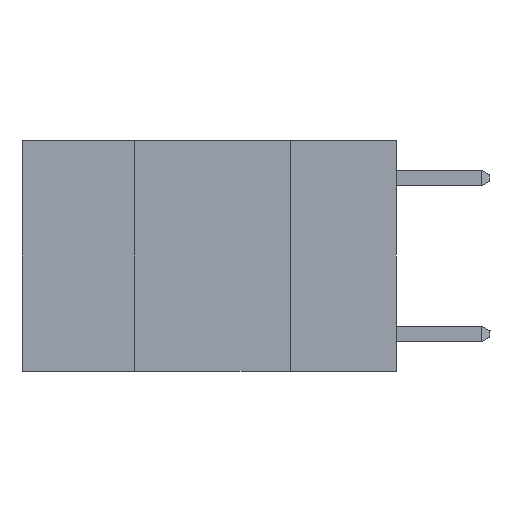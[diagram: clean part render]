
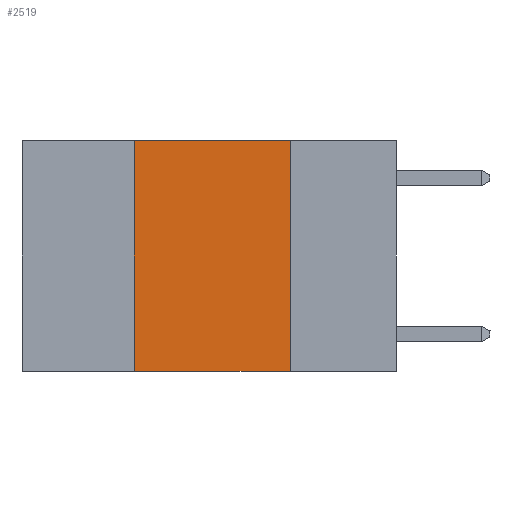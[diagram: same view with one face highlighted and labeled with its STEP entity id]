
A CAD part, left-side view. The second image highlights one B-rep face of the part: STEP entity #2519.
In plain terms, the highlighted planar face has unit normal (-1, 0, 0).
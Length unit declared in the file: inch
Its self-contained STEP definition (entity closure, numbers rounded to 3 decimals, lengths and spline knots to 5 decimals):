
#1854 = LINE ( 'NONE', #18751, #12563 ) ;
#1991 = ORIENTED_EDGE ( 'NONE', *, *, #6561, .F. ) ;
#2420 = ORIENTED_EDGE ( 'NONE', *, *, #10808, .F. ) ;
#2477 = ORIENTED_EDGE ( 'NONE', *, *, #16576, .F. ) ;
#2519 = ADVANCED_FACE ( 'NONE', ( #9225 ), #19426, .F. ) ;
#2618 = CARTESIAN_POINT ( 'NONE',  ( 0., 0.6, 0. ) ) ;
#3506 = ORIENTED_EDGE ( 'NONE', *, *, #18267, .T. ) ;
#4051 = CARTESIAN_POINT ( 'NONE',  ( 0., 0.42, 0. ) ) ;
#4134 = DIRECTION ( 'NONE',  ( 0., -1., 0. ) ) ;
#4524 = VECTOR ( 'NONE', #5489, 39.37008 ) ;
#5489 = DIRECTION ( 'NONE',  ( 0., 0., 1. ) ) ;
#6561 = EDGE_CURVE ( 'NONE', #18247, #21882, #13895, .T. ) ;
#6803 = LINE ( 'NONE', #7490, #11802 ) ;
#6926 = VECTOR ( 'NONE', #13787, 39.37008 ) ;
#6960 = DIRECTION ( 'NONE',  ( 1., 0., 0. ) ) ;
#7490 = CARTESIAN_POINT ( 'NONE',  ( 0., 0.17, 0. ) ) ;
#9003 = CARTESIAN_POINT ( 'NONE',  ( 0., 0.17, 0. ) ) ;
#9225 = FACE_OUTER_BOUND ( 'NONE', #10987, .T. ) ;
#9578 = DIRECTION ( 'NONE',  ( 0., 0., -1. ) ) ;
#10808 = EDGE_CURVE ( 'NONE', #21882, #12151, #6803, .T. ) ;
#10987 = EDGE_LOOP ( 'NONE', ( #2420, #1991, #2477, #3506 ) ) ;
#11802 = VECTOR ( 'NONE', #9578, 39.37008 ) ;
#12151 = VERTEX_POINT ( 'NONE', #19691 ) ;
#12563 = VECTOR ( 'NONE', #4134, 39.37008 ) ;
#13787 = DIRECTION ( 'NONE',  ( 0., -1., 0. ) ) ;
#13895 = LINE ( 'NONE', #25637, #6926 ) ;
#15053 = VERTEX_POINT ( 'NONE', #24981 ) ;
#15097 = LINE ( 'NONE', #21993, #4524 ) ;
#16576 = EDGE_CURVE ( 'NONE', #15053, #18247, #15097, .T. ) ;
#17855 = AXIS2_PLACEMENT_3D ( 'NONE', #2618, #6960, #21485 ) ;
#18247 = VERTEX_POINT ( 'NONE', #4051 ) ;
#18267 = EDGE_CURVE ( 'NONE', #15053, #12151, #1854, .T. ) ;
#18751 = CARTESIAN_POINT ( 'NONE',  ( 0., 0.6, -0.37 ) ) ;
#19426 = PLANE ( 'NONE',  #17855 ) ;
#19691 = CARTESIAN_POINT ( 'NONE',  ( 0., 0.17, -0.37 ) ) ;
#21485 = DIRECTION ( 'NONE',  ( 0., 0., -1. ) ) ;
#21882 = VERTEX_POINT ( 'NONE', #9003 ) ;
#21993 = CARTESIAN_POINT ( 'NONE',  ( 0., 0.42, 0. ) ) ;
#24981 = CARTESIAN_POINT ( 'NONE',  ( 0., 0.42, -0.37 ) ) ;
#25637 = CARTESIAN_POINT ( 'NONE',  ( 0., 0.6, 0. ) ) ;
